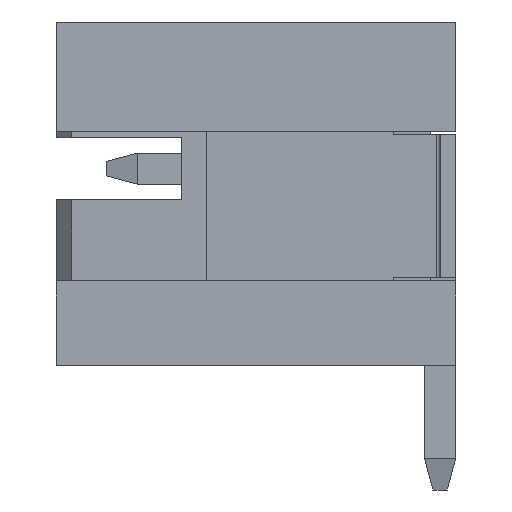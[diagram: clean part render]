
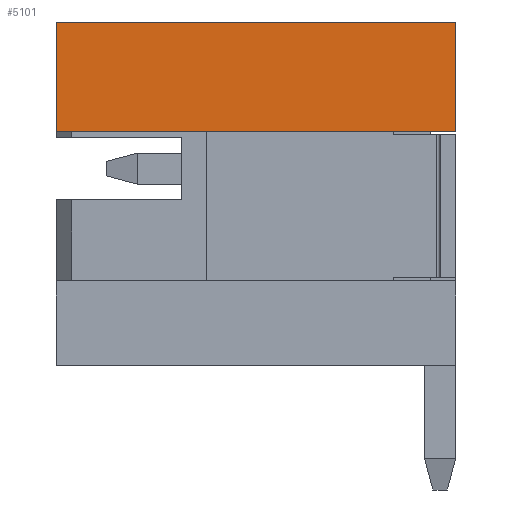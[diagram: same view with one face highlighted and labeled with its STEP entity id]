
A CAD part, left-side view. The second image highlights one B-rep face of the part: STEP entity #5101.
In plain terms, the highlighted planar face has unit normal (-1, 0, 0).
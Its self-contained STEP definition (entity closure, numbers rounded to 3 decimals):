
#56 = EDGE_CURVE ( 'NONE', #2378, #7913, #6680, .T. ) ;
#619 = EDGE_CURVE ( 'NONE', #7913, #5782, #1963, .T. ) ;
#1117 = ORIENTED_EDGE ( 'NONE', *, *, #56, .F. ) ;
#1197 = LINE ( 'NONE', #5909, #2188 ) ;
#1604 = DIRECTION ( 'NONE',  ( 0., 1., 0. ) ) ;
#1788 = EDGE_LOOP ( 'NONE', ( #5067, #5914, #1117, #5259 ) ) ;
#1963 = LINE ( 'NONE', #2371, #6251 ) ;
#2114 = DIRECTION ( 'NONE',  ( 0., 0., 1. ) ) ;
#2140 = CARTESIAN_POINT ( 'NONE',  ( -3., 0., 0.6 ) ) ;
#2188 = VECTOR ( 'NONE', #2114, 1000. ) ;
#2371 = CARTESIAN_POINT ( 'NONE',  ( -3., 0., 0.6 ) ) ;
#2378 = VERTEX_POINT ( 'NONE', #2897 ) ;
#2405 = VECTOR ( 'NONE', #6282, 1000. ) ;
#2536 = CARTESIAN_POINT ( 'NONE',  ( -3., 6.4, 0.6 ) ) ;
#2897 = CARTESIAN_POINT ( 'NONE',  ( -3., 0., 2.35 ) ) ;
#3201 = CARTESIAN_POINT ( 'NONE',  ( -3., 0., 0. ) ) ;
#3592 = CARTESIAN_POINT ( 'NONE',  ( -3., 6.4, 2.35 ) ) ;
#4095 = LINE ( 'NONE', #5692, #2405 ) ;
#4096 = VECTOR ( 'NONE', #5506, 1000. ) ;
#4191 = AXIS2_PLACEMENT_3D ( 'NONE', #3201, #4220, #7025 ) ;
#4220 = DIRECTION ( 'NONE',  ( 1., 0., 0. ) ) ;
#4297 = CARTESIAN_POINT ( 'NONE',  ( -3., 0., 2.35 ) ) ;
#4413 = PLANE ( 'NONE',  #4191 ) ;
#4676 = FACE_OUTER_BOUND ( 'NONE', #1788, .T. ) ;
#5067 = ORIENTED_EDGE ( 'NONE', *, *, #6095, .F. ) ;
#5101 = ADVANCED_FACE ( 'NONE', ( #4676 ), #4413, .F. ) ;
#5134 = EDGE_CURVE ( 'NONE', #6664, #2378, #4095, .T. ) ;
#5259 = ORIENTED_EDGE ( 'NONE', *, *, #5134, .F. ) ;
#5506 = DIRECTION ( 'NONE',  ( 0., 0., -1. ) ) ;
#5692 = CARTESIAN_POINT ( 'NONE',  ( -3., 6.4, 2.35 ) ) ;
#5782 = VERTEX_POINT ( 'NONE', #2536 ) ;
#5909 = CARTESIAN_POINT ( 'NONE',  ( -3., 6.4, 2.35 ) ) ;
#5914 = ORIENTED_EDGE ( 'NONE', *, *, #619, .F. ) ;
#6095 = EDGE_CURVE ( 'NONE', #5782, #6664, #1197, .T. ) ;
#6251 = VECTOR ( 'NONE', #1604, 1000. ) ;
#6282 = DIRECTION ( 'NONE',  ( 0., -1., 0. ) ) ;
#6664 = VERTEX_POINT ( 'NONE', #3592 ) ;
#6680 = LINE ( 'NONE', #4297, #4096 ) ;
#7025 = DIRECTION ( 'NONE',  ( 0., 0., -1. ) ) ;
#7913 = VERTEX_POINT ( 'NONE', #2140 ) ;
